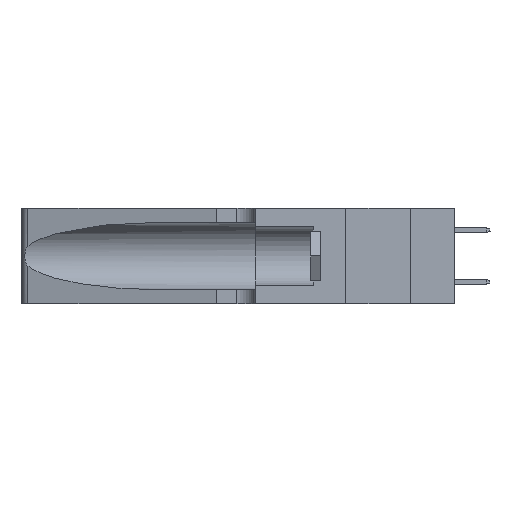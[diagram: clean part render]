
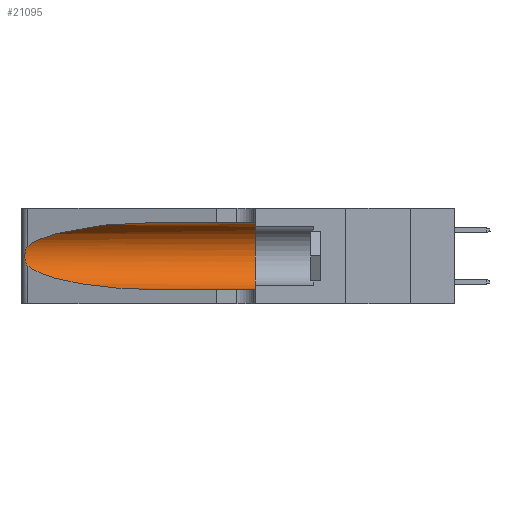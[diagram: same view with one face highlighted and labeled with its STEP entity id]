
A CAD part, left-side view. The second image highlights one B-rep face of the part: STEP entity #21095.
In plain terms, the highlighted cylindrical face has radius 3.308 mm (diameter 6.617 mm), a partial arc.
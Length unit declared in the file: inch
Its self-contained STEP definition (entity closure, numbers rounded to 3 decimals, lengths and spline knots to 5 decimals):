
#194 = EDGE_LOOP ( 'NONE', ( #43094, #41340, #26179, #37301, #37396, #15573 ) ) ;
#363 = CARTESIAN_POINT ( 'NONE',  ( 0.25787, 1.23484, 0.2124 ) ) ;
#1042 = CARTESIAN_POINT ( 'NONE',  ( 0.25856, 1.23593, 0.16098 ) ) ;
#1444 = FACE_OUTER_BOUND ( 'NONE', #194, .T. ) ;
#1926 = DIRECTION ( 'NONE',  ( 0., 0., 1. ) ) ;
#2908 =( BOUNDED_CURVE ( )  B_SPLINE_CURVE ( 3, ( #19217, #23544, #33159, #40868 ),
 .UNSPECIFIED., .F., .T. ) 
 B_SPLINE_CURVE_WITH_KNOTS ( ( 4, 4 ),
 ( 1.5708, 2.84003 ),
 .UNSPECIFIED. ) 
 CURVE ( )  GEOMETRIC_REPRESENTATION_ITEM ( )  RATIONAL_B_SPLINE_CURVE ( ( 1., 0.87, 0.87, 1. ) ) 
 REPRESENTATION_ITEM ( '' )  );
#2953 = EDGE_CURVE ( 'NONE', #23408, #4377, #23935, .T. ) ;
#4377 = VERTEX_POINT ( 'NONE', #36472 ) ;
#4479 = CARTESIAN_POINT ( 'NONE',  ( 0.25854, 1.2359, 0.20912 ) ) ;
#4708 = CARTESIAN_POINT ( 'NONE',  ( 0.25789, 1.23486, 0.15765 ) ) ;
#5333 = CARTESIAN_POINT ( 'NONE',  ( 0.1305, 1.61858, 0.185 ) ) ;
#6814 = CARTESIAN_POINT ( 'NONE',  ( 0.1305, 1.61858, 0.31525 ) ) ;
#7418 = VERTEX_POINT ( 'NONE', #21639 ) ;
#7457 = CARTESIAN_POINT ( 'NONE',  ( 0.25555, 1.22993, 0.14849 ) ) ;
#10869 = CARTESIAN_POINT ( 'NONE',  ( 0.25487, 1.22718, 0.14631 ) ) ;
#13363 = EDGE_CURVE ( 'NONE', #4377, #38506, #35283, .T. ) ;
#13397 = AXIS2_PLACEMENT_3D ( 'NONE', #43255, #19517, #1926 ) ;
#14071 = CARTESIAN_POINT ( 'NONE',  ( 0.1305, 0.72297, 0.05475 ) ) ;
#14285 = CARTESIAN_POINT ( 'NONE',  ( 0.2373, 1.15595, 0.08982 ) ) ;
#14302 = CARTESIAN_POINT ( 'NONE',  ( 0.26075, 1.23896, 0.178 ) ) ;
#15573 = ORIENTED_EDGE ( 'NONE', *, *, #2953, .F. ) ;
#15731 = VERTEX_POINT ( 'NONE', #22596 ) ;
#16484 = VECTOR ( 'NONE', #20747, 39.37008 ) ;
#16859 = CARTESIAN_POINT ( 'NONE',  ( 0.25487, 1.22718, 0.22369 ) ) ;
#17959 = CARTESIAN_POINT ( 'NONE',  ( 0.25639, 1.23184, 0.21858 ) ) ;
#19217 = CARTESIAN_POINT ( 'NONE',  ( 0.1305, 0.72297, 0.31525 ) ) ;
#19517 = DIRECTION ( 'NONE',  ( 0., 1., 0. ) ) ;
#20747 = DIRECTION ( 'NONE',  ( 0., -1., 0. ) ) ;
#21095 = ADVANCED_FACE ( 'NONE', ( #1444 ), #36394, .F. ) ;
#21325 =( BOUNDED_CURVE ( )  B_SPLINE_CURVE ( 3, ( #41918, #14285, #31436, #14071 ),
 .UNSPECIFIED., .F., .T. ) 
 B_SPLINE_CURVE_WITH_KNOTS ( ( 4, 4 ),
 ( 3.44316, 4.71239 ),
 .UNSPECIFIED. ) 
 CURVE ( )  GEOMETRIC_REPRESENTATION_ITEM ( )  RATIONAL_B_SPLINE_CURVE ( ( 1., 0.87, 0.87, 1. ) ) 
 REPRESENTATION_ITEM ( '' )  );
#21639 = CARTESIAN_POINT ( 'NONE',  ( 0.25487, 1.22718, 0.14631 ) ) ;
#22596 = CARTESIAN_POINT ( 'NONE',  ( 0.1305, 0.72297, 0.05475 ) ) ;
#23408 = VERTEX_POINT ( 'NONE', #40070 ) ;
#23544 = CARTESIAN_POINT ( 'NONE',  ( 0.18966, 0.96281, 0.31525 ) ) ;
#23935 = LINE ( 'NONE', #6814, #16484 ) ;
#24211 = CARTESIAN_POINT ( 'NONE',  ( 0.1305, 0.35, 0.05475 ) ) ;
#26068 = VERTEX_POINT ( 'NONE', #16859 ) ;
#26179 = ORIENTED_EDGE ( 'NONE', *, *, #30458, .T. ) ;
#26829 = EDGE_CURVE ( 'NONE', #23408, #26068, #2908, .T. ) ;
#28239 = CARTESIAN_POINT ( 'NONE',  ( 0.26017, 1.23833, 0.17102 ) ) ;
#28757 = CARTESIAN_POINT ( 'NONE',  ( 0.1305, 1.61858, 0.05475 ) ) ;
#29144 = CARTESIAN_POINT ( 'NONE',  ( 0.26075, 1.23896, 0.19203 ) ) ;
#30458 = EDGE_CURVE ( 'NONE', #7418, #15731, #21325, .T. ) ;
#31436 = CARTESIAN_POINT ( 'NONE',  ( 0.18966, 0.96281, 0.05475 ) ) ;
#31541 = EDGE_CURVE ( 'NONE', #26068, #7418, #45062, .T. ) ;
#31676 = CARTESIAN_POINT ( 'NONE',  ( 0.25555, 1.22994, 0.2215 ) ) ;
#32178 = LINE ( 'NONE', #28757, #40299 ) ;
#33159 = CARTESIAN_POINT ( 'NONE',  ( 0.2373, 1.15595, 0.28018 ) ) ;
#35283 = CIRCLE ( 'NONE', #13397, 0.13025 ) ;
#35768 = CARTESIAN_POINT ( 'NONE',  ( 0.25487, 1.22718, 0.22369 ) ) ;
#35990 = CARTESIAN_POINT ( 'NONE',  ( 0.26018, 1.23835, 0.19895 ) ) ;
#36394 = CYLINDRICAL_SURFACE ( 'NONE', #36538, 0.13025 ) ;
#36472 = CARTESIAN_POINT ( 'NONE',  ( 0.1305, 0.35, 0.31525 ) ) ;
#36538 = AXIS2_PLACEMENT_3D ( 'NONE', #5333, #36848, #43231 ) ;
#36848 = DIRECTION ( 'NONE',  ( 0., -1., 0. ) ) ;
#37294 = EDGE_CURVE ( 'NONE', #15731, #38506, #32178, .T. ) ;
#37301 = ORIENTED_EDGE ( 'NONE', *, *, #37294, .T. ) ;
#37396 = ORIENTED_EDGE ( 'NONE', *, *, #13363, .F. ) ;
#38506 = VERTEX_POINT ( 'NONE', #24211 ) ;
#38962 = CARTESIAN_POINT ( 'NONE',  ( 0.25639, 1.23186, 0.15144 ) ) ;
#40070 = CARTESIAN_POINT ( 'NONE',  ( 0.1305, 0.72297, 0.31525 ) ) ;
#40299 = VECTOR ( 'NONE', #42657, 39.37008 ) ;
#40868 = CARTESIAN_POINT ( 'NONE',  ( 0.25487, 1.22718, 0.22369 ) ) ;
#41340 = ORIENTED_EDGE ( 'NONE', *, *, #31541, .T. ) ;
#41918 = CARTESIAN_POINT ( 'NONE',  ( 0.25487, 1.22718, 0.14631 ) ) ;
#42657 = DIRECTION ( 'NONE',  ( 0., -1., 0. ) ) ;
#43094 = ORIENTED_EDGE ( 'NONE', *, *, #26829, .T. ) ;
#43231 = DIRECTION ( 'NONE',  ( 0., 0., -1. ) ) ;
#43255 = CARTESIAN_POINT ( 'NONE',  ( 0.1305, 0.35, 0.185 ) ) ;
#45062 = B_SPLINE_CURVE_WITH_KNOTS ( 'NONE', 3,
 ( #35768, #31676, #17959, #363, #4479, #35990, #29144, #14302, #28239, #1042, #4708, #38962, #7457, #10869 ),
 .UNSPECIFIED., .F., .F.,
 ( 4, 2, 2, 2, 2, 2, 4 ),
 ( 0., 0.00027, 0.00053, 0.00107, 0.0016, 0.00187, 0.00214 ),
 .UNSPECIFIED. ) ;
